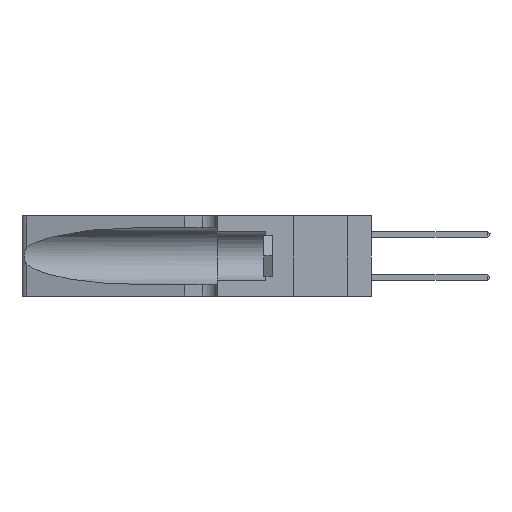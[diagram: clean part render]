
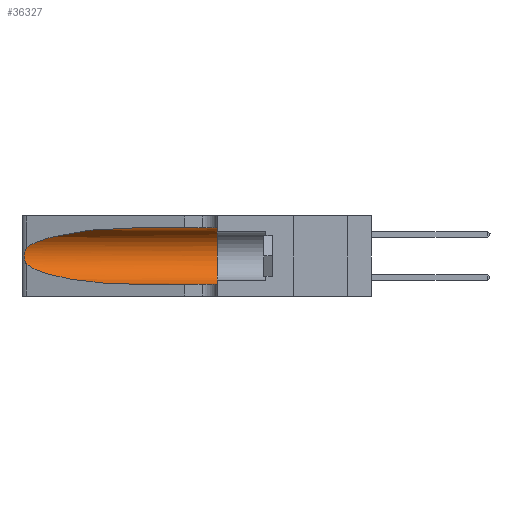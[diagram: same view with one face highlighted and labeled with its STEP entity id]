
A CAD part, left-side view. The second image highlights one B-rep face of the part: STEP entity #36327.
In plain terms, the highlighted cylindrical face has radius 3.308 mm (diameter 6.617 mm), a partial arc.
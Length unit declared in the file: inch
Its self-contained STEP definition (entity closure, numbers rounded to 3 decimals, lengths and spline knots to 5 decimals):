
#751 = EDGE_LOOP ( 'NONE', ( #24384, #21714, #38920, #4590, #9502, #32757 ) ) ;
#1484 = DIRECTION ( 'NONE',  ( 0., 1., 0. ) ) ;
#1567 = AXIS2_PLACEMENT_3D ( 'NONE', #23193, #1484, #42160 ) ;
#1900 = CARTESIAN_POINT ( 'NONE',  ( 0.18966, 0.96281, 0.31525 ) ) ;
#2551 = CARTESIAN_POINT ( 'NONE',  ( 0.25555, 1.22993, 0.14849 ) ) ;
#2671 = EDGE_CURVE ( 'NONE', #22566, #5858, #42394, .T. ) ;
#2704 = CARTESIAN_POINT ( 'NONE',  ( 0.25639, 1.23184, 0.21858 ) ) ;
#3019 = CARTESIAN_POINT ( 'NONE',  ( 0.25487, 1.22718, 0.22369 ) ) ;
#3394 = CIRCLE ( 'NONE', #1567, 0.13025 ) ;
#3675 = CARTESIAN_POINT ( 'NONE',  ( 0.25487, 1.22718, 0.14631 ) ) ;
#4590 = ORIENTED_EDGE ( 'NONE', *, *, #42477, .T. ) ;
#5839 = CARTESIAN_POINT ( 'NONE',  ( 0.25487, 1.22718, 0.22369 ) ) ;
#5858 = VERTEX_POINT ( 'NONE', #22403 ) ;
#6167 = CARTESIAN_POINT ( 'NONE',  ( 0.25487, 1.22718, 0.14631 ) ) ;
#6481 = CARTESIAN_POINT ( 'NONE',  ( 0.26018, 1.23835, 0.19895 ) ) ;
#8443 = DIRECTION ( 'NONE',  ( 0., -1., 0. ) ) ;
#8992 = CARTESIAN_POINT ( 'NONE',  ( 0.2373, 1.15595, 0.28018 ) ) ;
#9502 = ORIENTED_EDGE ( 'NONE', *, *, #30739, .F. ) ;
#10284 = CARTESIAN_POINT ( 'NONE',  ( 0.25555, 1.22994, 0.2215 ) ) ;
#11585 = LINE ( 'NONE', #16199, #16146 ) ;
#11588 =( BOUNDED_CURVE ( )  B_SPLINE_CURVE ( 3, ( #3675, #13789, #14245, #32037 ),
 .UNSPECIFIED., .F., .T. ) 
 B_SPLINE_CURVE_WITH_KNOTS ( ( 4, 4 ),
 ( 3.44316, 4.71239 ),
 .UNSPECIFIED. ) 
 CURVE ( )  GEOMETRIC_REPRESENTATION_ITEM ( )  RATIONAL_B_SPLINE_CURVE ( ( 1., 0.87, 0.87, 1. ) ) 
 REPRESENTATION_ITEM ( '' )  );
#13766 = CARTESIAN_POINT ( 'NONE',  ( 0.26075, 1.23896, 0.178 ) ) ;
#13789 = CARTESIAN_POINT ( 'NONE',  ( 0.2373, 1.15595, 0.08982 ) ) ;
#14245 = CARTESIAN_POINT ( 'NONE',  ( 0.18966, 0.96281, 0.05475 ) ) ;
#15832 = DIRECTION ( 'NONE',  ( 0., -1., 0. ) ) ;
#16146 = VECTOR ( 'NONE', #8443, 39.37008 ) ;
#16199 = CARTESIAN_POINT ( 'NONE',  ( 0.1305, 1.61858, 0.31525 ) ) ;
#16669 = EDGE_CURVE ( 'NONE', #44859, #32725, #11588, .T. ) ;
#19968 = LINE ( 'NONE', #26373, #34691 ) ;
#20027 = B_SPLINE_CURVE_WITH_KNOTS ( 'NONE', 3,
 ( #3019, #10284, #2704, #38786, #42931, #6481, #20737, #13766, #39099, #28059, #38627, #46142, #2551, #6167 ),
 .UNSPECIFIED., .F., .F.,
 ( 4, 2, 2, 2, 2, 2, 4 ),
 ( 0., 0.00027, 0.00053, 0.00107, 0.0016, 0.00187, 0.00214 ),
 .UNSPECIFIED. ) ;
#20737 = CARTESIAN_POINT ( 'NONE',  ( 0.26075, 1.23896, 0.19203 ) ) ;
#21714 = ORIENTED_EDGE ( 'NONE', *, *, #22557, .T. ) ;
#21773 = AXIS2_PLACEMENT_3D ( 'NONE', #29806, #15832, #44376 ) ;
#22293 = CARTESIAN_POINT ( 'NONE',  ( 0.1305, 0.35, 0.31525 ) ) ;
#22403 = CARTESIAN_POINT ( 'NONE',  ( 0.25487, 1.22718, 0.22369 ) ) ;
#22557 = EDGE_CURVE ( 'NONE', #5858, #44859, #20027, .T. ) ;
#22566 = VERTEX_POINT ( 'NONE', #31695 ) ;
#23193 = CARTESIAN_POINT ( 'NONE',  ( 0.1305, 0.35, 0.185 ) ) ;
#24384 = ORIENTED_EDGE ( 'NONE', *, *, #2671, .T. ) ;
#26373 = CARTESIAN_POINT ( 'NONE',  ( 0.1305, 1.61858, 0.05475 ) ) ;
#28059 = CARTESIAN_POINT ( 'NONE',  ( 0.25856, 1.23593, 0.16098 ) ) ;
#29546 = FACE_OUTER_BOUND ( 'NONE', #751, .T. ) ;
#29806 = CARTESIAN_POINT ( 'NONE',  ( 0.1305, 1.61858, 0.185 ) ) ;
#30739 = EDGE_CURVE ( 'NONE', #36863, #32309, #3394, .T. ) ;
#31180 = CARTESIAN_POINT ( 'NONE',  ( 0.1305, 0.72297, 0.05475 ) ) ;
#31695 = CARTESIAN_POINT ( 'NONE',  ( 0.1305, 0.72297, 0.31525 ) ) ;
#32037 = CARTESIAN_POINT ( 'NONE',  ( 0.1305, 0.72297, 0.05475 ) ) ;
#32309 = VERTEX_POINT ( 'NONE', #46305 ) ;
#32725 = VERTEX_POINT ( 'NONE', #31180 ) ;
#32757 = ORIENTED_EDGE ( 'NONE', *, *, #40971, .F. ) ;
#33786 = DIRECTION ( 'NONE',  ( 0., -1., 0. ) ) ;
#34691 = VECTOR ( 'NONE', #33786, 39.37008 ) ;
#36327 = ADVANCED_FACE ( 'NONE', ( #29546 ), #37444, .F. ) ;
#36863 = VERTEX_POINT ( 'NONE', #22293 ) ;
#37444 = CYLINDRICAL_SURFACE ( 'NONE', #21773, 0.13025 ) ;
#38627 = CARTESIAN_POINT ( 'NONE',  ( 0.25789, 1.23486, 0.15765 ) ) ;
#38786 = CARTESIAN_POINT ( 'NONE',  ( 0.25787, 1.23484, 0.2124 ) ) ;
#38920 = ORIENTED_EDGE ( 'NONE', *, *, #16669, .T. ) ;
#39099 = CARTESIAN_POINT ( 'NONE',  ( 0.26017, 1.23833, 0.17102 ) ) ;
#39971 = CARTESIAN_POINT ( 'NONE',  ( 0.25487, 1.22718, 0.14631 ) ) ;
#40971 = EDGE_CURVE ( 'NONE', #22566, #36863, #11585, .T. ) ;
#41928 = CARTESIAN_POINT ( 'NONE',  ( 0.1305, 0.72297, 0.31525 ) ) ;
#42160 = DIRECTION ( 'NONE',  ( 0., 0., 1. ) ) ;
#42394 =( BOUNDED_CURVE ( )  B_SPLINE_CURVE ( 3, ( #41928, #1900, #8992, #5839 ),
 .UNSPECIFIED., .F., .T. ) 
 B_SPLINE_CURVE_WITH_KNOTS ( ( 4, 4 ),
 ( 1.5708, 2.84003 ),
 .UNSPECIFIED. ) 
 CURVE ( )  GEOMETRIC_REPRESENTATION_ITEM ( )  RATIONAL_B_SPLINE_CURVE ( ( 1., 0.87, 0.87, 1. ) ) 
 REPRESENTATION_ITEM ( '' )  );
#42477 = EDGE_CURVE ( 'NONE', #32725, #32309, #19968, .T. ) ;
#42931 = CARTESIAN_POINT ( 'NONE',  ( 0.25854, 1.2359, 0.20912 ) ) ;
#44376 = DIRECTION ( 'NONE',  ( 0., 0., -1. ) ) ;
#44859 = VERTEX_POINT ( 'NONE', #39971 ) ;
#46142 = CARTESIAN_POINT ( 'NONE',  ( 0.25639, 1.23186, 0.15144 ) ) ;
#46305 = CARTESIAN_POINT ( 'NONE',  ( 0.1305, 0.35, 0.05475 ) ) ;
